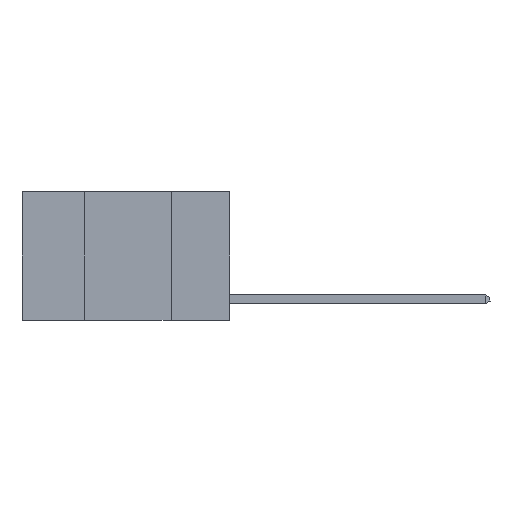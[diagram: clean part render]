
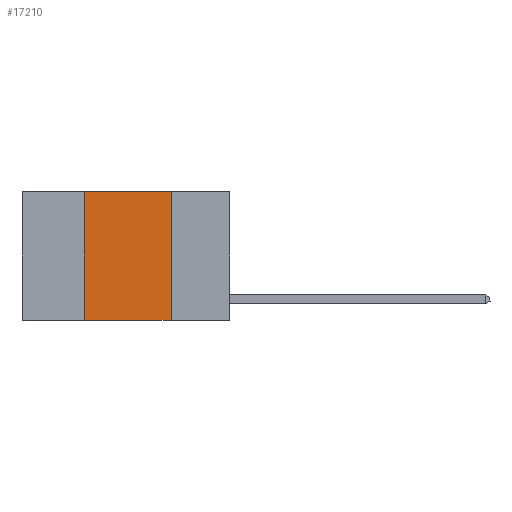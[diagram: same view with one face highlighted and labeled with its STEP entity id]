
A CAD part, left-side view. The second image highlights one B-rep face of the part: STEP entity #17210.
In plain terms, the highlighted planar face has unit normal (-1, 0, 0).
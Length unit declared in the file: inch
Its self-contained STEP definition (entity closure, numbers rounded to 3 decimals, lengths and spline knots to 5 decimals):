
#3665 = DIRECTION ( 'NONE',  ( 1., 0., 0. ) ) ;
#3701 = CARTESIAN_POINT ( 'NONE',  ( 0., 0.17, 0. ) ) ;
#4286 = LINE ( 'NONE', #6787, #13789 ) ;
#4459 = VERTEX_POINT ( 'NONE', #16989 ) ;
#4563 = DIRECTION ( 'NONE',  ( 0., 0., 1. ) ) ;
#6017 = LINE ( 'NONE', #16678, #8736 ) ;
#6084 = VERTEX_POINT ( 'NONE', #11144 ) ;
#6138 = CARTESIAN_POINT ( 'NONE',  ( 0., 0.42, 0. ) ) ;
#6279 = CARTESIAN_POINT ( 'NONE',  ( 0., 0.6, -0.37 ) ) ;
#6787 = CARTESIAN_POINT ( 'NONE',  ( 0., 0.6, 0. ) ) ;
#7247 = VECTOR ( 'NONE', #18961, 39.37008 ) ;
#8160 = CARTESIAN_POINT ( 'NONE',  ( 0., 0.42, 0. ) ) ;
#8163 = VECTOR ( 'NONE', #4563, 39.37008 ) ;
#8736 = VECTOR ( 'NONE', #18401, 39.37008 ) ;
#9163 = EDGE_LOOP ( 'NONE', ( #15579, #12812, #13768, #14258 ) ) ;
#10022 = DIRECTION ( 'NONE',  ( 0., -1., 0. ) ) ;
#10210 = EDGE_CURVE ( 'NONE', #15464, #6084, #6017, .T. ) ;
#10715 = FACE_OUTER_BOUND ( 'NONE', #9163, .T. ) ;
#11144 = CARTESIAN_POINT ( 'NONE',  ( 0., 0.17, -0.37 ) ) ;
#12761 = VERTEX_POINT ( 'NONE', #8160 ) ;
#12812 = ORIENTED_EDGE ( 'NONE', *, *, #15550, .F. ) ;
#12892 = EDGE_CURVE ( 'NONE', #4459, #12761, #14360, .T. ) ;
#13768 = ORIENTED_EDGE ( 'NONE', *, *, #12892, .F. ) ;
#13789 = VECTOR ( 'NONE', #10022, 39.37008 ) ;
#14258 = ORIENTED_EDGE ( 'NONE', *, *, #17451, .T. ) ;
#14360 = LINE ( 'NONE', #6138, #8163 ) ;
#14825 = DIRECTION ( 'NONE',  ( 0., 0., -1. ) ) ;
#15464 = VERTEX_POINT ( 'NONE', #3701 ) ;
#15550 = EDGE_CURVE ( 'NONE', #12761, #15464, #4286, .T. ) ;
#15579 = ORIENTED_EDGE ( 'NONE', *, *, #10210, .F. ) ;
#16678 = CARTESIAN_POINT ( 'NONE',  ( 0., 0.17, 0. ) ) ;
#16989 = CARTESIAN_POINT ( 'NONE',  ( 0., 0.42, -0.37 ) ) ;
#17210 = ADVANCED_FACE ( 'NONE', ( #10715 ), #17589, .F. ) ;
#17451 = EDGE_CURVE ( 'NONE', #4459, #6084, #19404, .T. ) ;
#17589 = PLANE ( 'NONE',  #20579 ) ;
#18401 = DIRECTION ( 'NONE',  ( 0., 0., -1. ) ) ;
#18961 = DIRECTION ( 'NONE',  ( 0., -1., 0. ) ) ;
#19232 = CARTESIAN_POINT ( 'NONE',  ( 0., 0.6, 0. ) ) ;
#19404 = LINE ( 'NONE', #6279, #7247 ) ;
#20579 = AXIS2_PLACEMENT_3D ( 'NONE', #19232, #3665, #14825 ) ;
